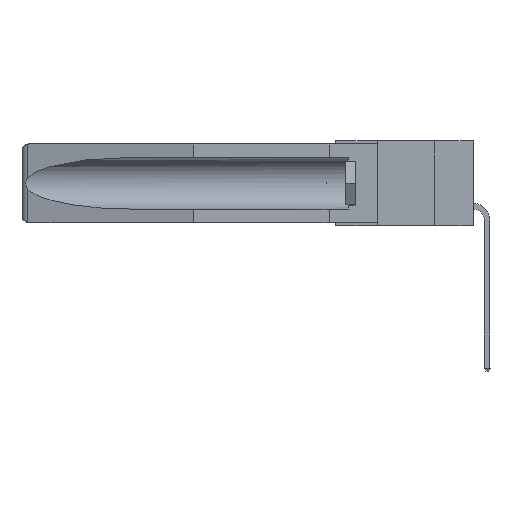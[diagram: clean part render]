
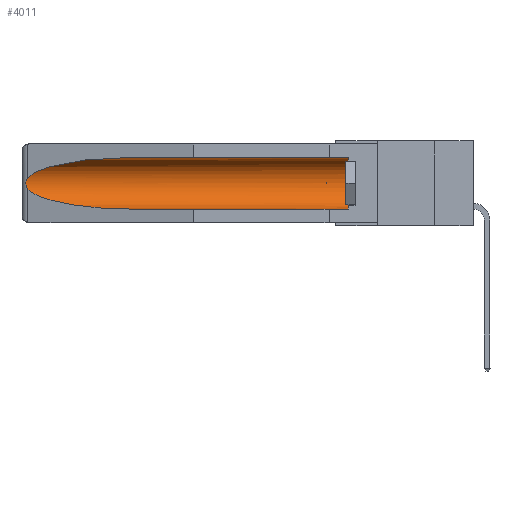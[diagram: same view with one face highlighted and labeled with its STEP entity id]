
A CAD part, left-side view. The second image highlights one B-rep face of the part: STEP entity #4011.
In plain terms, the highlighted cylindrical face has radius 2.857 mm (diameter 5.715 mm), a partial arc.
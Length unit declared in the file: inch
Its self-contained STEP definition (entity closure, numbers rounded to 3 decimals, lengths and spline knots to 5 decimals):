
#279 = FACE_OUTER_BOUND ( 'NONE', #1177, .T. ) ;
#336 = CARTESIAN_POINT ( 'NONE',  ( 0.155, 0.126, -0.284 ) ) ;
#1177 = EDGE_LOOP ( 'NONE', ( #29746, #2774, #10476, #26861, #10670, #27412 ) ) ;
#1868 = CARTESIAN_POINT ( 'NONE',  ( 0.155, -0.30754, -0.284 ) ) ;
#2508 = CARTESIAN_POINT ( 'NONE',  ( 0.2673, 1.5327, -0.16383 ) ) ;
#2737 = CARTESIAN_POINT ( 'NONE',  ( 0.21114, 1.30732, -0.059 ) ) ;
#2774 = ORIENTED_EDGE ( 'NONE', *, *, #13705, .T. ) ;
#2837 = CARTESIAN_POINT ( 'NONE',  ( 0.26537, 1.52718, -0.19328 ) ) ;
#3082 = CARTESIAN_POINT ( 'NONE',  ( 0.26537, 1.52718, -0.14972 ) ) ;
#3327 = EDGE_CURVE ( 'NONE', #29274, #22899, #14324, .T. ) ;
#4011 = ADVANCED_FACE ( 'NONE', ( #279 ), #8435, .F. ) ;
#4051 = AXIS2_PLACEMENT_3D ( 'NONE', #21182, #10772, #15823 ) ;
#4264 = CARTESIAN_POINT ( 'NONE',  ( 0.155, 1.07973, -0.059 ) ) ;
#4356 = EDGE_CURVE ( 'NONE', #5988, #22899, #15777, .T. ) ;
#5124 = CARTESIAN_POINT ( 'NONE',  ( 0.2675, 1.53308, -0.17534 ) ) ;
#5341 = CARTESIAN_POINT ( 'NONE',  ( 0.25451, 1.48313, -0.09465 ) ) ;
#5988 = VERTEX_POINT ( 'NONE', #336 ) ;
#6921 = CARTESIAN_POINT ( 'NONE',  ( 0.21114, 1.30732, -0.284 ) ) ;
#7827 = VECTOR ( 'NONE', #23849, 39.37008 ) ;
#8232 = B_SPLINE_CURVE_WITH_KNOTS ( 'NONE', 3,
 ( #18508, #18396, #26289, #2508, #10598, #5124, #10709, #26072, #28791, #2837 ),
 .UNSPECIFIED., .F., .F.,
 ( 4, 2, 2, 2, 4 ),
 ( 0., 0.00029, 0.00058, 0.00087, 0.00117 ),
 .UNSPECIFIED. ) ;
#8402 = VECTOR ( 'NONE', #28243, 39.37008 ) ;
#8435 = CYLINDRICAL_SURFACE ( 'NONE', #4051, 0.1125 ) ;
#9130 = CARTESIAN_POINT ( 'NONE',  ( 0.26537, 1.52718, -0.19328 ) ) ;
#9253 = VERTEX_POINT ( 'NONE', #22429 ) ;
#10476 = ORIENTED_EDGE ( 'NONE', *, *, #3327, .T. ) ;
#10523 = EDGE_CURVE ( 'NONE', #19879, #22891, #24589, .T. ) ;
#10598 = CARTESIAN_POINT ( 'NONE',  ( 0.2675, 1.53308, -0.16763 ) ) ;
#10670 = ORIENTED_EDGE ( 'NONE', *, *, #21068, .T. ) ;
#10699 = CARTESIAN_POINT ( 'NONE',  ( 0.155, -0.30754, -0.059 ) ) ;
#10709 = CARTESIAN_POINT ( 'NONE',  ( 0.2673, 1.53269, -0.17917 ) ) ;
#10772 = DIRECTION ( 'NONE',  ( 0., 1., 0. ) ) ;
#11971 = CARTESIAN_POINT ( 'NONE',  ( 0.25451, 1.48313, -0.24835 ) ) ;
#12128 = EDGE_CURVE ( 'NONE', #9253, #19879, #33675, .T. ) ;
#13705 = EDGE_CURVE ( 'NONE', #22891, #29274, #8232, .T. ) ;
#14324 =( BOUNDED_CURVE ( )  B_SPLINE_CURVE ( 3, ( #9130, #11971, #6921, #24916 ),
 .UNSPECIFIED., .F., .F. ) 
 B_SPLINE_CURVE_WITH_KNOTS ( ( 4, 4 ),
 ( 0.1948, 1.5708 ),
 .UNSPECIFIED. ) 
 CURVE ( )  GEOMETRIC_REPRESENTATION_ITEM ( )  RATIONAL_B_SPLINE_CURVE ( ( 1., 0.848, 0.848, 1. ) ) 
 REPRESENTATION_ITEM ( '' )  );
#15777 = LINE ( 'NONE', #1868, #8402 ) ;
#15823 = DIRECTION ( 'NONE',  ( 0., 0., 1. ) ) ;
#16450 = CARTESIAN_POINT ( 'NONE',  ( 0.155, 1.07973, -0.284 ) ) ;
#17219 = DIRECTION ( 'NONE',  ( 0., 0., 1. ) ) ;
#18396 = CARTESIAN_POINT ( 'NONE',  ( 0.26597, 1.52961, -0.15275 ) ) ;
#18508 = CARTESIAN_POINT ( 'NONE',  ( 0.26537, 1.52718, -0.14972 ) ) ;
#19057 = CARTESIAN_POINT ( 'NONE',  ( 0.155, 0.126, -0.1715 ) ) ;
#19879 = VERTEX_POINT ( 'NONE', #4264 ) ;
#21068 = EDGE_CURVE ( 'NONE', #5988, #9253, #33282, .T. ) ;
#21182 = CARTESIAN_POINT ( 'NONE',  ( 0.155, -0.30754, -0.1715 ) ) ;
#21351 = CARTESIAN_POINT ( 'NONE',  ( 0.26537, 1.52718, -0.14972 ) ) ;
#21995 = CARTESIAN_POINT ( 'NONE',  ( 0.26537, 1.52718, -0.19328 ) ) ;
#22429 = CARTESIAN_POINT ( 'NONE',  ( 0.155, 0.126, -0.059 ) ) ;
#22572 = DIRECTION ( 'NONE',  ( 0., -1., 0. ) ) ;
#22891 = VERTEX_POINT ( 'NONE', #3082 ) ;
#22899 = VERTEX_POINT ( 'NONE', #16450 ) ;
#23849 = DIRECTION ( 'NONE',  ( 0., 1., 0. ) ) ;
#24589 =( BOUNDED_CURVE ( )  B_SPLINE_CURVE ( 3, ( #28797, #2737, #5341, #21351 ),
 .UNSPECIFIED., .F., .F. ) 
 B_SPLINE_CURVE_WITH_KNOTS ( ( 4, 4 ),
 ( 4.71239, 6.08839 ),
 .UNSPECIFIED. ) 
 CURVE ( )  GEOMETRIC_REPRESENTATION_ITEM ( )  RATIONAL_B_SPLINE_CURVE ( ( 1., 0.848, 0.848, 1. ) ) 
 REPRESENTATION_ITEM ( '' )  );
#24916 = CARTESIAN_POINT ( 'NONE',  ( 0.155, 1.07973, -0.284 ) ) ;
#26072 = CARTESIAN_POINT ( 'NONE',  ( 0.26655, 1.53094, -0.18657 ) ) ;
#26289 = CARTESIAN_POINT ( 'NONE',  ( 0.26654, 1.53092, -0.15636 ) ) ;
#26861 = ORIENTED_EDGE ( 'NONE', *, *, #4356, .F. ) ;
#27412 = ORIENTED_EDGE ( 'NONE', *, *, #12128, .T. ) ;
#27596 = AXIS2_PLACEMENT_3D ( 'NONE', #19057, #22572, #17219 ) ;
#28243 = DIRECTION ( 'NONE',  ( 0., 1., 0. ) ) ;
#28791 = CARTESIAN_POINT ( 'NONE',  ( 0.26597, 1.5296, -0.19026 ) ) ;
#28797 = CARTESIAN_POINT ( 'NONE',  ( 0.155, 1.07973, -0.059 ) ) ;
#29274 = VERTEX_POINT ( 'NONE', #21995 ) ;
#29746 = ORIENTED_EDGE ( 'NONE', *, *, #10523, .T. ) ;
#33282 = CIRCLE ( 'NONE', #27596, 0.1125 ) ;
#33675 = LINE ( 'NONE', #10699, #7827 ) ;
